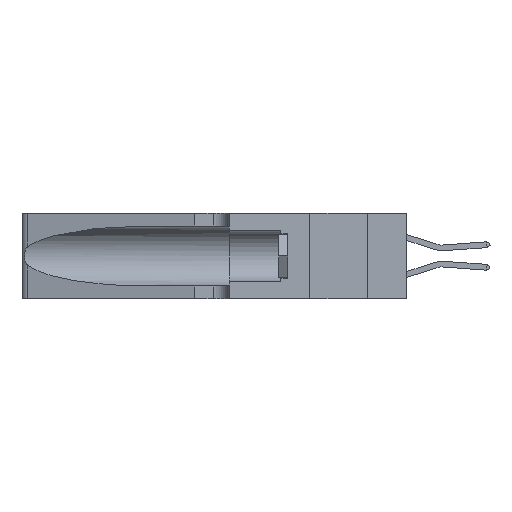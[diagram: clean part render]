
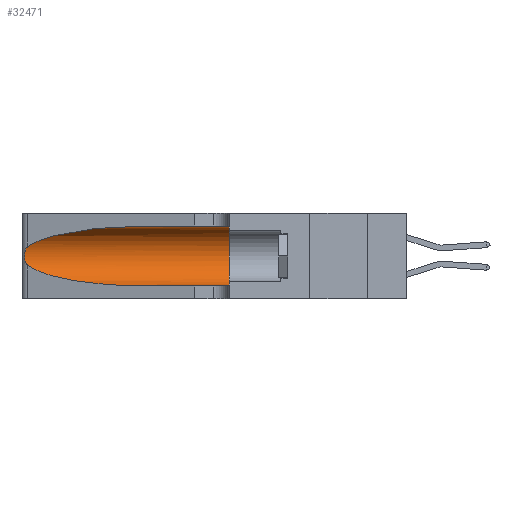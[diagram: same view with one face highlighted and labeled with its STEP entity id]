
A CAD part, left-side view. The second image highlights one B-rep face of the part: STEP entity #32471.
In plain terms, the highlighted cylindrical face has radius 3.308 mm (diameter 6.617 mm), a partial arc.
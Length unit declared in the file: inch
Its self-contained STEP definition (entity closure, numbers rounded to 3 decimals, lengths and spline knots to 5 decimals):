
#604 = DIRECTION ( 'NONE',  ( 0., 0., -1. ) ) ;
#637 = CARTESIAN_POINT ( 'NONE',  ( 0.18966, 0.96281, 0.31525 ) ) ;
#1031 =( BOUNDED_CURVE ( )  B_SPLINE_CURVE ( 3, ( #9738, #12992, #35142, #16191 ),
 .UNSPECIFIED., .F., .F. ) 
 B_SPLINE_CURVE_WITH_KNOTS ( ( 4, 4 ),
 ( 3.44316, 4.71239 ),
 .UNSPECIFIED. ) 
 CURVE ( )  GEOMETRIC_REPRESENTATION_ITEM ( )  RATIONAL_B_SPLINE_CURVE ( ( 1., 0.87, 0.87, 1. ) ) 
 REPRESENTATION_ITEM ( '' )  );
#1830 = CARTESIAN_POINT ( 'NONE',  ( 0.25487, 1.22718, 0.14631 ) ) ;
#3563 = VERTEX_POINT ( 'NONE', #36750 ) ;
#3564 = CARTESIAN_POINT ( 'NONE',  ( 0.1305, 1.61858, 0.05475 ) ) ;
#3900 = CARTESIAN_POINT ( 'NONE',  ( 0.2373, 1.15595, 0.28018 ) ) ;
#4541 = DIRECTION ( 'NONE',  ( 0., 1., 0. ) ) ;
#4969 = CARTESIAN_POINT ( 'NONE',  ( 0.25639, 1.23184, 0.21858 ) ) ;
#6864 = DIRECTION ( 'NONE',  ( 0., -1., 0. ) ) ;
#6889 = CARTESIAN_POINT ( 'NONE',  ( 0.25487, 1.22718, 0.22369 ) ) ;
#8238 = CARTESIAN_POINT ( 'NONE',  ( 0.25854, 1.2359, 0.20912 ) ) ;
#8559 = ORIENTED_EDGE ( 'NONE', *, *, #29163, .F. ) ;
#9089 = LINE ( 'NONE', #3564, #33472 ) ;
#9366 = CIRCLE ( 'NONE', #16077, 0.13025 ) ;
#9738 = CARTESIAN_POINT ( 'NONE',  ( 0.25487, 1.22718, 0.14631 ) ) ;
#10044 = EDGE_CURVE ( 'NONE', #20221, #16002, #23489, .T. ) ;
#10650 = EDGE_CURVE ( 'NONE', #3563, #23408, #9089, .T. ) ;
#10859 = VERTEX_POINT ( 'NONE', #33148 ) ;
#10901 = EDGE_CURVE ( 'NONE', #16002, #10859, #16087, .T. ) ;
#11485 = CARTESIAN_POINT ( 'NONE',  ( 0.26075, 1.23896, 0.19203 ) ) ;
#12455 = CARTESIAN_POINT ( 'NONE',  ( 0.1305, 1.61858, 0.31525 ) ) ;
#12992 = CARTESIAN_POINT ( 'NONE',  ( 0.2373, 1.15595, 0.08982 ) ) ;
#14301 = ORIENTED_EDGE ( 'NONE', *, *, #23445, .F. ) ;
#14674 = CYLINDRICAL_SURFACE ( 'NONE', #30142, 0.13025 ) ;
#14735 = CARTESIAN_POINT ( 'NONE',  ( 0.26017, 1.23833, 0.17102 ) ) ;
#15132 = CARTESIAN_POINT ( 'NONE',  ( 0.1305, 0.35, 0.31525 ) ) ;
#15458 = ORIENTED_EDGE ( 'NONE', *, *, #10901, .T. ) ;
#15751 = ORIENTED_EDGE ( 'NONE', *, *, #27267, .T. ) ;
#16002 = VERTEX_POINT ( 'NONE', #6889 ) ;
#16077 = AXIS2_PLACEMENT_3D ( 'NONE', #23785, #4541, #26977 ) ;
#16087 = B_SPLINE_CURVE_WITH_KNOTS ( 'NONE', 3,
 ( #20981, #24192, #4969, #27388, #8238, #30562, #11485, #33704, #14735, #36806, #17885, #39936, #21125, #1830 ),
 .UNSPECIFIED., .F., .F.,
 ( 4, 2, 2, 2, 2, 2, 4 ),
 ( 0., 0.00027, 0.00053, 0.00107, 0.0016, 0.00187, 0.00214 ),
 .UNSPECIFIED. ) ;
#16191 = CARTESIAN_POINT ( 'NONE',  ( 0.1305, 0.72297, 0.05475 ) ) ;
#17885 = CARTESIAN_POINT ( 'NONE',  ( 0.25789, 1.23486, 0.15765 ) ) ;
#19336 = CARTESIAN_POINT ( 'NONE',  ( 0.1305, 0.72297, 0.31525 ) ) ;
#19894 = CARTESIAN_POINT ( 'NONE',  ( 0.1305, 1.61858, 0.185 ) ) ;
#20027 = EDGE_LOOP ( 'NONE', ( #27985, #15458, #15751, #23946, #14301, #8559 ) ) ;
#20221 = VERTEX_POINT ( 'NONE', #19336 ) ;
#20428 = LINE ( 'NONE', #12455, #35257 ) ;
#20981 = CARTESIAN_POINT ( 'NONE',  ( 0.25487, 1.22718, 0.22369 ) ) ;
#21125 = CARTESIAN_POINT ( 'NONE',  ( 0.25555, 1.22993, 0.14849 ) ) ;
#23167 = CARTESIAN_POINT ( 'NONE',  ( 0.1305, 0.72297, 0.31525 ) ) ;
#23408 = VERTEX_POINT ( 'NONE', #23652 ) ;
#23445 = EDGE_CURVE ( 'NONE', #26539, #23408, #9366, .T. ) ;
#23489 =( BOUNDED_CURVE ( )  B_SPLINE_CURVE ( 3, ( #23167, #637, #3900, #26357 ),
 .UNSPECIFIED., .F., .F. ) 
 B_SPLINE_CURVE_WITH_KNOTS ( ( 4, 4 ),
 ( 1.5708, 2.84003 ),
 .UNSPECIFIED. ) 
 CURVE ( )  GEOMETRIC_REPRESENTATION_ITEM ( )  RATIONAL_B_SPLINE_CURVE ( ( 1., 0.87, 0.87, 1. ) ) 
 REPRESENTATION_ITEM ( '' )  );
#23652 = CARTESIAN_POINT ( 'NONE',  ( 0.1305, 0.35, 0.05475 ) ) ;
#23785 = CARTESIAN_POINT ( 'NONE',  ( 0.1305, 0.35, 0.185 ) ) ;
#23946 = ORIENTED_EDGE ( 'NONE', *, *, #10650, .T. ) ;
#24192 = CARTESIAN_POINT ( 'NONE',  ( 0.25555, 1.22994, 0.2215 ) ) ;
#26357 = CARTESIAN_POINT ( 'NONE',  ( 0.25487, 1.22718, 0.22369 ) ) ;
#26539 = VERTEX_POINT ( 'NONE', #15132 ) ;
#26977 = DIRECTION ( 'NONE',  ( 0., 0., 1. ) ) ;
#27267 = EDGE_CURVE ( 'NONE', #10859, #3563, #1031, .T. ) ;
#27388 = CARTESIAN_POINT ( 'NONE',  ( 0.25787, 1.23484, 0.2124 ) ) ;
#27985 = ORIENTED_EDGE ( 'NONE', *, *, #10044, .T. ) ;
#29163 = EDGE_CURVE ( 'NONE', #20221, #26539, #20428, .T. ) ;
#30142 = AXIS2_PLACEMENT_3D ( 'NONE', #19894, #32504, #604 ) ;
#30562 = CARTESIAN_POINT ( 'NONE',  ( 0.26018, 1.23835, 0.19895 ) ) ;
#31553 = FACE_OUTER_BOUND ( 'NONE', #20027, .T. ) ;
#32471 = ADVANCED_FACE ( 'NONE', ( #31553 ), #14674, .F. ) ;
#32504 = DIRECTION ( 'NONE',  ( 0., -1., 0. ) ) ;
#33148 = CARTESIAN_POINT ( 'NONE',  ( 0.25487, 1.22718, 0.14631 ) ) ;
#33472 = VECTOR ( 'NONE', #6864, 39.37008 ) ;
#33704 = CARTESIAN_POINT ( 'NONE',  ( 0.26075, 1.23896, 0.178 ) ) ;
#35142 = CARTESIAN_POINT ( 'NONE',  ( 0.18966, 0.96281, 0.05475 ) ) ;
#35257 = VECTOR ( 'NONE', #37751, 39.37008 ) ;
#36750 = CARTESIAN_POINT ( 'NONE',  ( 0.1305, 0.72297, 0.05475 ) ) ;
#36806 = CARTESIAN_POINT ( 'NONE',  ( 0.25856, 1.23593, 0.16098 ) ) ;
#37751 = DIRECTION ( 'NONE',  ( 0., -1., 0. ) ) ;
#39936 = CARTESIAN_POINT ( 'NONE',  ( 0.25639, 1.23186, 0.15144 ) ) ;
